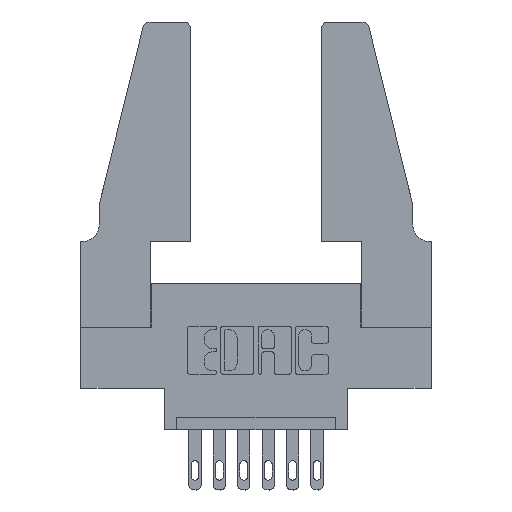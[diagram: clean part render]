
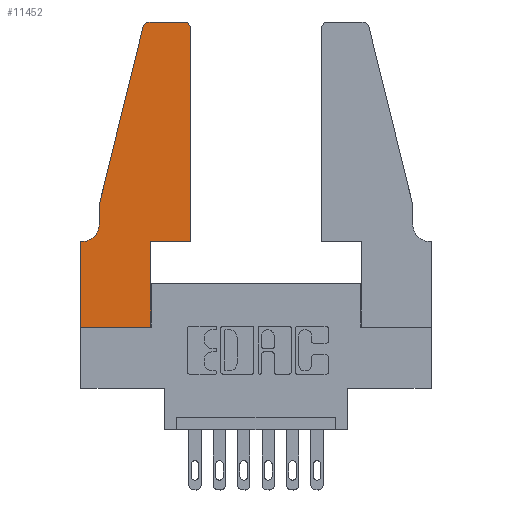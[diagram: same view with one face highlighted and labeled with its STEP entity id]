
A CAD part, top view. The second image highlights one B-rep face of the part: STEP entity #11452.
In plain terms, the highlighted planar face has unit normal (0, 0, 1).
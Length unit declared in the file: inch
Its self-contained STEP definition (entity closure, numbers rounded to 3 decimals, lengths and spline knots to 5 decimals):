
#1 = LINE ( 'NONE', #2521, #9211 ) ;
#17 = EDGE_CURVE ( 'NONE', #6732, #8760, #1, .T. ) ;
#28 = CARTESIAN_POINT ( 'NONE',  ( 0.4505, 1.22, 0.37 ) ) ;
#97 = DIRECTION ( 'NONE',  ( 1., 0., 0. ) ) ;
#219 = VECTOR ( 'NONE', #7377, 39.37008 ) ;
#223 = VERTEX_POINT ( 'NONE', #3830 ) ;
#664 = DIRECTION ( 'NONE',  ( 0., 0., 1. ) ) ;
#809 = ORIENTED_EDGE ( 'NONE', *, *, #8898, .T. ) ;
#914 = FACE_OUTER_BOUND ( 'NONE', #7744, .T. ) ;
#1190 = ORIENTED_EDGE ( 'NONE', *, *, #5954, .T. ) ;
#1472 = PLANE ( 'NONE',  #4944 ) ;
#1474 = EDGE_CURVE ( 'NONE', #5858, #3222, #11014, .T. ) ;
#1604 = DIRECTION ( 'NONE',  ( -1., 0., 0. ) ) ;
#1738 = LINE ( 'NONE', #7334, #219 ) ;
#1857 = CARTESIAN_POINT ( 'NONE',  ( 0.284, 1.22, 0.37 ) ) ;
#2021 = DIRECTION ( 'NONE',  ( 0., 1., 0. ) ) ;
#2024 = DIRECTION ( 'NONE',  ( 1., 0., 0. ) ) ;
#2052 = CARTESIAN_POINT ( 'NONE',  ( 0.4505, 0.35, 0.37 ) ) ;
#2152 = VECTOR ( 'NONE', #2021, 39.37008 ) ;
#2217 = CIRCLE ( 'NONE', #6505, 0.07 ) ;
#2488 = VECTOR ( 'NONE', #1604, 39.37008 ) ;
#2521 = CARTESIAN_POINT ( 'NONE',  ( 0.4505, 0.35, 0.37 ) ) ;
#2539 = EDGE_CURVE ( 'NONE', #3688, #8435, #2902, .T. ) ;
#2660 = DIRECTION ( 'NONE',  ( 0., 0., 1. ) ) ;
#2800 = DIRECTION ( 'NONE',  ( 0., 0., 1. ) ) ;
#2902 = LINE ( 'NONE', #6039, #2488 ) ;
#3125 = VECTOR ( 'NONE', #5001, 39.37008 ) ;
#3222 = VERTEX_POINT ( 'NONE', #3513 ) ;
#3409 = ORIENTED_EDGE ( 'NONE', *, *, #17, .T. ) ;
#3513 = CARTESIAN_POINT ( 'NONE',  ( 0.0755, 0.42, 0.37 ) ) ;
#3566 = VECTOR ( 'NONE', #8674, 39.37008 ) ;
#3593 = DIRECTION ( 'NONE',  ( 0., 1., 0. ) ) ;
#3638 = EDGE_CURVE ( 'NONE', #11201, #3688, #6568, .T. ) ;
#3688 = VERTEX_POINT ( 'NONE', #6483 ) ;
#3701 = EDGE_CURVE ( 'NONE', #8435, #9997, #10695, .T. ) ;
#3770 = CARTESIAN_POINT ( 'NONE',  ( 0., 0., 0.37 ) ) ;
#3830 = CARTESIAN_POINT ( 'NONE',  ( 0.0055, 0.35, 0.37 ) ) ;
#3859 = ORIENTED_EDGE ( 'NONE', *, *, #9381, .T. ) ;
#4126 = CARTESIAN_POINT ( 'NONE',  ( 0.2865, 0., 0.37 ) ) ;
#4168 = CARTESIAN_POINT ( 'NONE',  ( 0.0755, 0.5, 0.37 ) ) ;
#4393 = DIRECTION ( 'NONE',  ( 1., 0., 0. ) ) ;
#4516 = ORIENTED_EDGE ( 'NONE', *, *, #2539, .T. ) ;
#4710 = ORIENTED_EDGE ( 'NONE', *, *, #10780, .T. ) ;
#4863 = DIRECTION ( 'NONE',  ( -1., 0., 0. ) ) ;
#4874 = ORIENTED_EDGE ( 'NONE', *, *, #1474, .T. ) ;
#4944 = AXIS2_PLACEMENT_3D ( 'NONE', #7730, #664, #7695 ) ;
#4967 = CARTESIAN_POINT ( 'NONE',  ( 0.0755, 0.35, 0.37 ) ) ;
#5001 = DIRECTION ( 'NONE',  ( -0.239, -0.971, 0. ) ) ;
#5267 = CARTESIAN_POINT ( 'NONE',  ( 0.4205, 1.22, 0.37 ) ) ;
#5392 = LINE ( 'NONE', #3770, #8063 ) ;
#5435 = CARTESIAN_POINT ( 'NONE',  ( 0.284, 1.25, 0.37 ) ) ;
#5517 = CARTESIAN_POINT ( 'NONE',  ( 0., 0., 0.37 ) ) ;
#5521 = LINE ( 'NONE', #4168, #3125 ) ;
#5686 = ORIENTED_EDGE ( 'NONE', *, *, #3638, .T. ) ;
#5711 = DIRECTION ( 'NONE',  ( 0., 0., -1. ) ) ;
#5858 = VERTEX_POINT ( 'NONE', #8369 ) ;
#5954 = EDGE_CURVE ( 'NONE', #9550, #9011, #5392, .T. ) ;
#6039 = CARTESIAN_POINT ( 'NONE',  ( 0.2605, 1.25, 0.37 ) ) ;
#6149 = DIRECTION ( 'NONE',  ( 1., 0., 0. ) ) ;
#6483 = CARTESIAN_POINT ( 'NONE',  ( 0.4205, 1.25, 0.37 ) ) ;
#6505 = AXIS2_PLACEMENT_3D ( 'NONE', #6519, #5711, #4863 ) ;
#6519 = CARTESIAN_POINT ( 'NONE',  ( 0.0055, 0.42, 0.37 ) ) ;
#6568 = CIRCLE ( 'NONE', #6635, 0.03 ) ;
#6635 = AXIS2_PLACEMENT_3D ( 'NONE', #5267, #2660, #4393 ) ;
#6732 = VERTEX_POINT ( 'NONE', #10729 ) ;
#6735 = CARTESIAN_POINT ( 'NONE',  ( 0.25487, 1.22718, 0.37 ) ) ;
#6794 = ORIENTED_EDGE ( 'NONE', *, *, #3701, .T. ) ;
#7334 = CARTESIAN_POINT ( 'NONE',  ( 0., 0., 0.37 ) ) ;
#7377 = DIRECTION ( 'NONE',  ( 0., -1., 0. ) ) ;
#7466 = AXIS2_PLACEMENT_3D ( 'NONE', #1857, #2800, #97 ) ;
#7695 = DIRECTION ( 'NONE',  ( 1., 0., 0. ) ) ;
#7730 = CARTESIAN_POINT ( 'NONE',  ( 0., 0.35, 0.37 ) ) ;
#7744 = EDGE_LOOP ( 'NONE', ( #4516, #6794, #10608, #4874, #7983, #809, #7881, #1190, #3859, #3409, #4710, #5686 ) ) ;
#7788 = LINE ( 'NONE', #2052, #2152 ) ;
#7881 = ORIENTED_EDGE ( 'NONE', *, *, #11567, .T. ) ;
#7983 = ORIENTED_EDGE ( 'NONE', *, *, #8328, .T. ) ;
#8063 = VECTOR ( 'NONE', #2024, 39.37008 ) ;
#8328 = EDGE_CURVE ( 'NONE', #3222, #223, #2217, .T. ) ;
#8369 = CARTESIAN_POINT ( 'NONE',  ( 0.0755, 0.5, 0.37 ) ) ;
#8435 = VERTEX_POINT ( 'NONE', #5435 ) ;
#8674 = DIRECTION ( 'NONE',  ( 0., -1., 0. ) ) ;
#8760 = VERTEX_POINT ( 'NONE', #10607 ) ;
#8898 = EDGE_CURVE ( 'NONE', #223, #10633, #10077, .T. ) ;
#8947 = LINE ( 'NONE', #9652, #9080 ) ;
#9011 = VERTEX_POINT ( 'NONE', #4126 ) ;
#9080 = VECTOR ( 'NONE', #3593, 39.37008 ) ;
#9211 = VECTOR ( 'NONE', #6149, 39.37008 ) ;
#9381 = EDGE_CURVE ( 'NONE', #9011, #6732, #8947, .T. ) ;
#9550 = VERTEX_POINT ( 'NONE', #5517 ) ;
#9652 = CARTESIAN_POINT ( 'NONE',  ( 0.2865, 0.35, 0.37 ) ) ;
#9997 = VERTEX_POINT ( 'NONE', #6735 ) ;
#10077 = LINE ( 'NONE', #4967, #11322 ) ;
#10331 = CARTESIAN_POINT ( 'NONE',  ( 0., 0.35, 0.37 ) ) ;
#10409 = CARTESIAN_POINT ( 'NONE',  ( 0.0755, 0.5, 0.37 ) ) ;
#10607 = CARTESIAN_POINT ( 'NONE',  ( 0.4505, 0.35, 0.37 ) ) ;
#10608 = ORIENTED_EDGE ( 'NONE', *, *, #10712, .T. ) ;
#10633 = VERTEX_POINT ( 'NONE', #10331 ) ;
#10695 = CIRCLE ( 'NONE', #7466, 0.03 ) ;
#10712 = EDGE_CURVE ( 'NONE', #9997, #5858, #5521, .T. ) ;
#10729 = CARTESIAN_POINT ( 'NONE',  ( 0.2865, 0.35, 0.37 ) ) ;
#10780 = EDGE_CURVE ( 'NONE', #8760, #11201, #7788, .T. ) ;
#11014 = LINE ( 'NONE', #10409, #3566 ) ;
#11136 = DIRECTION ( 'NONE',  ( -1., 0., 0. ) ) ;
#11201 = VERTEX_POINT ( 'NONE', #28 ) ;
#11322 = VECTOR ( 'NONE', #11136, 39.37008 ) ;
#11452 = ADVANCED_FACE ( 'NONE', ( #914 ), #1472, .T. ) ;
#11567 = EDGE_CURVE ( 'NONE', #10633, #9550, #1738, .T. ) ;
